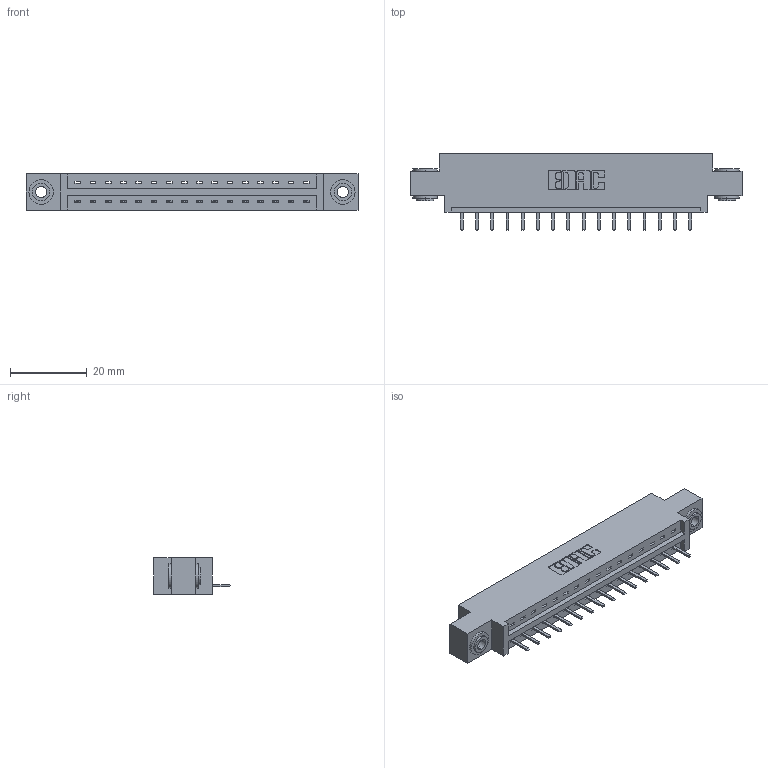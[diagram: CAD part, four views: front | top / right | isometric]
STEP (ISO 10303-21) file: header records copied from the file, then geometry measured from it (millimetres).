
FILE_DESCRIPTION (( 'STEP AP203' ), '1' );
FILE_NAME ('337-016-520-603.STEP', '2018-08-04T18:08:04', ( '' ), ( '' ), 'SwSTEP 2.0', 'SolidWorks 2016', '' );
FILE_SCHEMA (( 'CONFIG_CONTROL_DESIGN' ));
Length unit declared in the file: inch
Products named in the file (4): 337 Part_0.170 Offset - 0.156 Dia-TH; 345-292-001_345-293-120; 345-250-002_345-250-002-102; 337-016-520-603
Assembly tree (19 placements, depth 2):
  337-016-520-603
    337 Part_0.170 Offset - 0.156 Dia-TH
    345-292-001_345-293-120  x16
    345-250-002_345-250-002-102  x2
Bounding box: 86.41 x 20.02 x 9.4 mm (x, y, z)
Volume: 8511.5 mm3; surface area: 8814.5 mm2
Topology: 19 solids, 19 shells, 1212 faces, 3535 edges, 2310 vertices
Faces by surface type: plane 852, cylinder 352, cone 8
Entity records: 16152 total; most frequent: CARTESIAN_POINT 2801, ORIENTED_EDGE 2734, DIRECTION 2433, EDGE_CURVE 1367, LINE 1211, VECTOR 1211, VERTEX_POINT 906, AXIS2_PLACEMENT_3D 611
